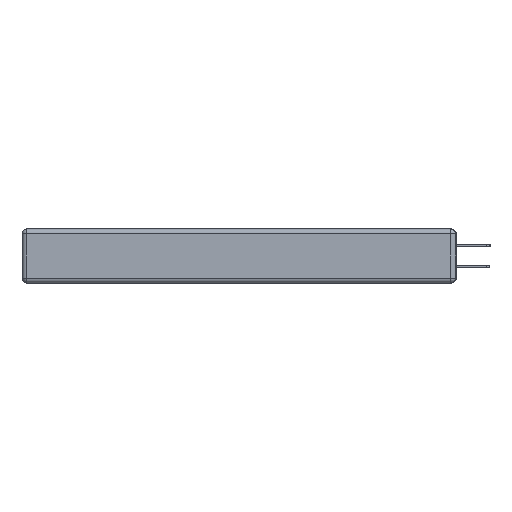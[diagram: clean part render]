
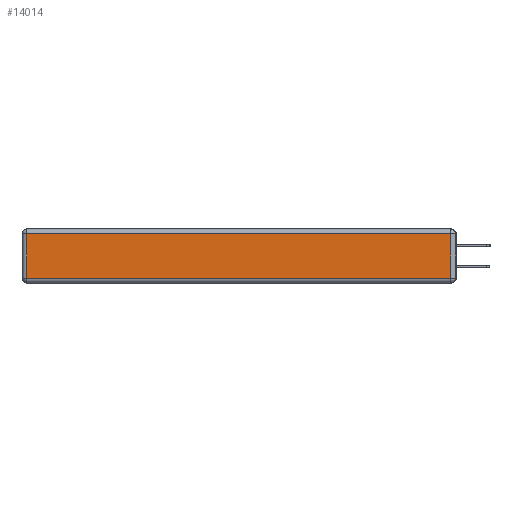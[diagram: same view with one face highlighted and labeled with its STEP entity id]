
A CAD part, left-side view. The second image highlights one B-rep face of the part: STEP entity #14014.
In plain terms, the highlighted planar face has unit normal (-1, 0, 0).
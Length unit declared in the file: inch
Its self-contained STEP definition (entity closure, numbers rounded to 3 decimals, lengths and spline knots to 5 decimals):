
#149 = DIRECTION ( 'NONE',  ( 0., 0., 1. ) ) ;
#310 = CARTESIAN_POINT ( 'NONE',  ( 0., 0.03, -0.343 ) ) ;
#1162 = CARTESIAN_POINT ( 'NONE',  ( 0., 2.72, -0.343 ) ) ;
#1868 = LINE ( 'NONE', #1162, #22112 ) ;
#2706 = VERTEX_POINT ( 'NONE', #22900 ) ;
#2981 = DIRECTION ( 'NONE',  ( 0., 1., 0. ) ) ;
#3567 = EDGE_LOOP ( 'NONE', ( #10788, #20679, #3883, #13733 ) ) ;
#3598 = CARTESIAN_POINT ( 'NONE',  ( 0., 2.72, -0.03 ) ) ;
#3883 = ORIENTED_EDGE ( 'NONE', *, *, #21528, .T. ) ;
#7275 = VECTOR ( 'NONE', #10214, 39.37008 ) ;
#7618 = DIRECTION ( 'NONE',  ( -1., 0., 0. ) ) ;
#9968 = CARTESIAN_POINT ( 'NONE',  ( 0., 0., -0.313 ) ) ;
#10214 = DIRECTION ( 'NONE',  ( 0., -1., 0. ) ) ;
#10325 = LINE ( 'NONE', #310, #13361 ) ;
#10566 = CARTESIAN_POINT ( 'NONE',  ( 0., 2.72, -0.313 ) ) ;
#10788 = ORIENTED_EDGE ( 'NONE', *, *, #15671, .T. ) ;
#12438 = VERTEX_POINT ( 'NONE', #3598 ) ;
#13361 = VECTOR ( 'NONE', #149, 39.37008 ) ;
#13416 = FACE_OUTER_BOUND ( 'NONE', #3567, .T. ) ;
#13691 = PLANE ( 'NONE',  #19955 ) ;
#13733 = ORIENTED_EDGE ( 'NONE', *, *, #14957, .T. ) ;
#14014 = ADVANCED_FACE ( 'NONE', ( #13416 ), #13691, .T. ) ;
#14618 = VERTEX_POINT ( 'NONE', #23956 ) ;
#14957 = EDGE_CURVE ( 'NONE', #12438, #20986, #1868, .T. ) ;
#15284 = EDGE_CURVE ( 'NONE', #2706, #14618, #10325, .T. ) ;
#15476 = VECTOR ( 'NONE', #2981, 39.37008 ) ;
#15562 = CARTESIAN_POINT ( 'NONE',  ( 0., 0., -0.343 ) ) ;
#15671 = EDGE_CURVE ( 'NONE', #20986, #2706, #16338, .T. ) ;
#16338 = LINE ( 'NONE', #9968, #7275 ) ;
#18348 = DIRECTION ( 'NONE',  ( 0., 0., -1. ) ) ;
#19459 = DIRECTION ( 'NONE',  ( 0., 0., 1. ) ) ;
#19955 = AXIS2_PLACEMENT_3D ( 'NONE', #15562, #7618, #19459 ) ;
#20276 = CARTESIAN_POINT ( 'NONE',  ( 0., 2.75, -0.03 ) ) ;
#20617 = LINE ( 'NONE', #20276, #15476 ) ;
#20679 = ORIENTED_EDGE ( 'NONE', *, *, #15284, .T. ) ;
#20986 = VERTEX_POINT ( 'NONE', #10566 ) ;
#21528 = EDGE_CURVE ( 'NONE', #14618, #12438, #20617, .T. ) ;
#22112 = VECTOR ( 'NONE', #18348, 39.37008 ) ;
#22900 = CARTESIAN_POINT ( 'NONE',  ( 0., 0.03, -0.313 ) ) ;
#23956 = CARTESIAN_POINT ( 'NONE',  ( 0., 0.03, -0.03 ) ) ;
